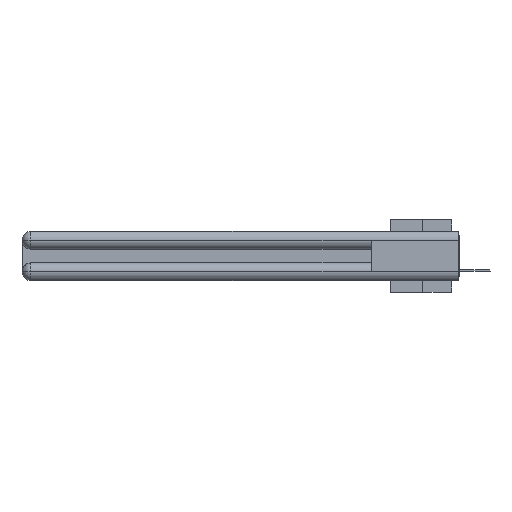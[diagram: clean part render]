
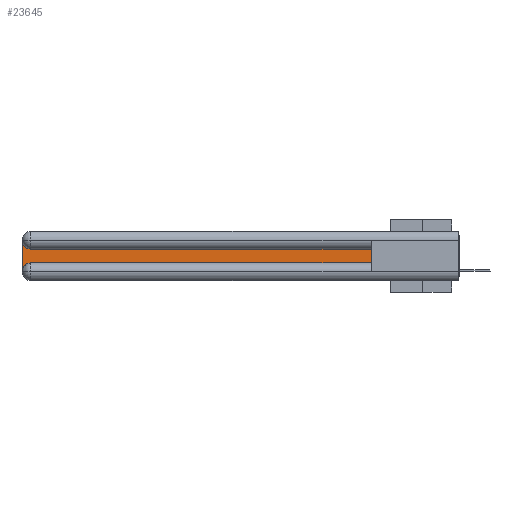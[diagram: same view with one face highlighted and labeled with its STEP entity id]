
A CAD part, left-side view. The second image highlights one B-rep face of the part: STEP entity #23645.
In plain terms, the highlighted planar face has unit normal (-1, 0, 0).
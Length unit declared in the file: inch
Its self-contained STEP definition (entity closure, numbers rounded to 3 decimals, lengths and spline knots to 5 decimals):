
#639 = CIRCLE ( 'NONE', #27228, 0.06 ) ;
#1416 = VECTOR ( 'NONE', #16349, 39.37008 ) ;
#1612 = CARTESIAN_POINT ( 'NONE',  ( 0.075, 0.6, -0.2175 ) ) ;
#1795 = LINE ( 'NONE', #7546, #25802 ) ;
#2214 = ORIENTED_EDGE ( 'NONE', *, *, #13345, .T. ) ;
#2236 = EDGE_LOOP ( 'NONE', ( #13271, #7304, #2214, #9628, #5704, #12185 ) ) ;
#3743 = VERTEX_POINT ( 'NONE', #15928 ) ;
#3848 = DIRECTION ( 'NONE',  ( 0., -1., 0. ) ) ;
#5336 = VERTEX_POINT ( 'NONE', #21357 ) ;
#5489 = AXIS2_PLACEMENT_3D ( 'NONE', #14527, #28902, #16881 ) ;
#5628 = DIRECTION ( 'NONE',  ( 1., 0., 0. ) ) ;
#5704 = ORIENTED_EDGE ( 'NONE', *, *, #8980, .T. ) ;
#7285 = CIRCLE ( 'NONE', #5489, 0.06 ) ;
#7304 = ORIENTED_EDGE ( 'NONE', *, *, #29121, .T. ) ;
#7546 = CARTESIAN_POINT ( 'NONE',  ( 0.075, 3., -0.2175 ) ) ;
#8017 = DIRECTION ( 'NONE',  ( 1., 0., 0. ) ) ;
#8980 = EDGE_CURVE ( 'NONE', #25953, #5336, #26516, .T. ) ;
#9312 = CARTESIAN_POINT ( 'NONE',  ( 0.075, 0.6, -0.1225 ) ) ;
#9628 = ORIENTED_EDGE ( 'NONE', *, *, #10612, .T. ) ;
#10015 = CARTESIAN_POINT ( 'NONE',  ( 0.075, 2.94, -0.2775 ) ) ;
#10061 = CARTESIAN_POINT ( 'NONE',  ( 0.075, 3., -0.0625 ) ) ;
#10359 = VERTEX_POINT ( 'NONE', #10061 ) ;
#10388 = DIRECTION ( 'NONE',  ( 0., 0., -1. ) ) ;
#10612 = EDGE_CURVE ( 'NONE', #29571, #25953, #639, .T. ) ;
#12185 = ORIENTED_EDGE ( 'NONE', *, *, #29402, .T. ) ;
#12691 = FACE_OUTER_BOUND ( 'NONE', #2236, .T. ) ;
#13271 = ORIENTED_EDGE ( 'NONE', *, *, #24623, .T. ) ;
#13345 = EDGE_CURVE ( 'NONE', #10359, #29571, #1795, .T. ) ;
#13639 = VECTOR ( 'NONE', #3848, 39.37008 ) ;
#14141 = LINE ( 'NONE', #9312, #15239 ) ;
#14527 = CARTESIAN_POINT ( 'NONE',  ( 0.075, 2.94, -0.0625 ) ) ;
#15239 = VECTOR ( 'NONE', #19346, 39.37008 ) ;
#15928 = CARTESIAN_POINT ( 'NONE',  ( 0.075, 2.94, -0.1225 ) ) ;
#16349 = DIRECTION ( 'NONE',  ( 0., 0., 1. ) ) ;
#16518 = LINE ( 'NONE', #1612, #1416 ) ;
#16881 = DIRECTION ( 'NONE',  ( 0., 0., -1. ) ) ;
#19346 = DIRECTION ( 'NONE',  ( 0., 1., 0. ) ) ;
#19771 = DIRECTION ( 'NONE',  ( 0., 0., -1. ) ) ;
#21221 = CARTESIAN_POINT ( 'NONE',  ( 0.075, 3., -0.2775 ) ) ;
#21357 = CARTESIAN_POINT ( 'NONE',  ( 0.075, 0.6, -0.2175 ) ) ;
#21370 = CARTESIAN_POINT ( 'NONE',  ( 0.075, 0.6, -0.1225 ) ) ;
#23645 = ADVANCED_FACE ( 'NONE', ( #12691 ), #24330, .F. ) ;
#24195 = CARTESIAN_POINT ( 'NONE',  ( 0.075, 2.94, -0.2175 ) ) ;
#24330 = PLANE ( 'NONE',  #27111 ) ;
#24623 = EDGE_CURVE ( 'NONE', #30071, #3743, #14141, .T. ) ;
#25802 = VECTOR ( 'NONE', #28771, 39.37008 ) ;
#25953 = VERTEX_POINT ( 'NONE', #24195 ) ;
#26516 = LINE ( 'NONE', #27627, #13639 ) ;
#27004 = CARTESIAN_POINT ( 'NONE',  ( 0.075, 3., -0.1225 ) ) ;
#27111 = AXIS2_PLACEMENT_3D ( 'NONE', #27004, #8017, #10388 ) ;
#27228 = AXIS2_PLACEMENT_3D ( 'NONE', #10015, #5628, #19771 ) ;
#27627 = CARTESIAN_POINT ( 'NONE',  ( 0.075, 0.6, -0.2175 ) ) ;
#28771 = DIRECTION ( 'NONE',  ( 0., 0., -1. ) ) ;
#28902 = DIRECTION ( 'NONE',  ( 1., 0., 0. ) ) ;
#29121 = EDGE_CURVE ( 'NONE', #3743, #10359, #7285, .T. ) ;
#29402 = EDGE_CURVE ( 'NONE', #5336, #30071, #16518, .T. ) ;
#29571 = VERTEX_POINT ( 'NONE', #21221 ) ;
#30071 = VERTEX_POINT ( 'NONE', #21370 ) ;
